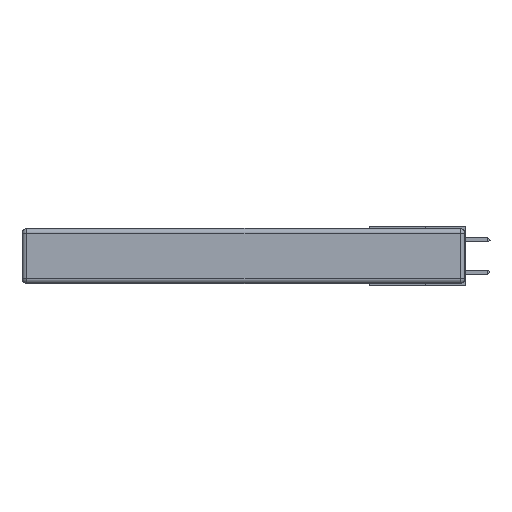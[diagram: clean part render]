
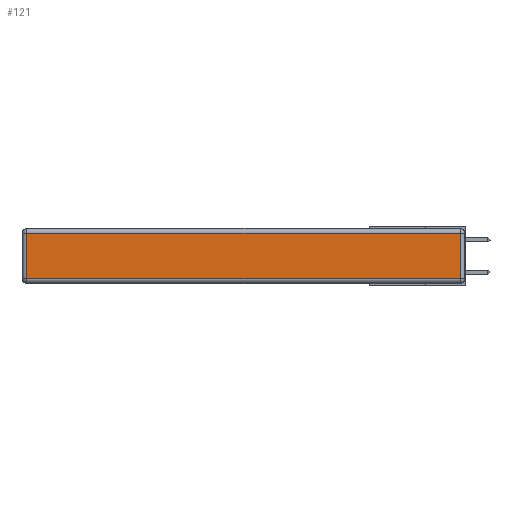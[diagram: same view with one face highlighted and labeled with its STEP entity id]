
A CAD part, left-side view. The second image highlights one B-rep face of the part: STEP entity #121.
In plain terms, the highlighted planar face has unit normal (-1, 0, 0).
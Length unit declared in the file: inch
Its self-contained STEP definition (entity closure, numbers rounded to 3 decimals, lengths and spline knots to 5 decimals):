
#121 = ADVANCED_FACE ( 'NONE', ( #670 ), #27151, .T. ) ;
#344 = VECTOR ( 'NONE', #29191, 39.37008 ) ;
#670 = FACE_OUTER_BOUND ( 'NONE', #27722, .T. ) ;
#856 = ORIENTED_EDGE ( 'NONE', *, *, #28431, .T. ) ;
#2791 = LINE ( 'NONE', #25806, #3155 ) ;
#3155 = VECTOR ( 'NONE', #28676, 39.37008 ) ;
#3933 = ORIENTED_EDGE ( 'NONE', *, *, #28927, .T. ) ;
#4337 = VERTEX_POINT ( 'NONE', #24066 ) ;
#5254 = CARTESIAN_POINT ( 'NONE',  ( 0., 2.72, -0.343 ) ) ;
#5694 = VECTOR ( 'NONE', #30632, 39.37008 ) ;
#6085 = VERTEX_POINT ( 'NONE', #6592 ) ;
#6592 = CARTESIAN_POINT ( 'NONE',  ( 0., 2.72, -0.03 ) ) ;
#6788 = CARTESIAN_POINT ( 'NONE',  ( 0., 0.03, -0.03 ) ) ;
#7111 = CARTESIAN_POINT ( 'NONE',  ( 0., 0., -0.343 ) ) ;
#13802 = VECTOR ( 'NONE', #24035, 39.37008 ) ;
#13983 = EDGE_CURVE ( 'NONE', #6085, #19820, #27896, .T. ) ;
#16495 = EDGE_CURVE ( 'NONE', #4337, #17255, #25729, .T. ) ;
#17074 = AXIS2_PLACEMENT_3D ( 'NONE', #7111, #26930, #17117 ) ;
#17117 = DIRECTION ( 'NONE',  ( 0., 0., 1. ) ) ;
#17255 = VERTEX_POINT ( 'NONE', #6788 ) ;
#19820 = VERTEX_POINT ( 'NONE', #32250 ) ;
#21319 = ORIENTED_EDGE ( 'NONE', *, *, #16495, .T. ) ;
#21330 = CARTESIAN_POINT ( 'NONE',  ( 0., 0., -0.313 ) ) ;
#24035 = DIRECTION ( 'NONE',  ( 0., -1., 0. ) ) ;
#24066 = CARTESIAN_POINT ( 'NONE',  ( 0., 0.03, -0.313 ) ) ;
#25358 = ORIENTED_EDGE ( 'NONE', *, *, #13983, .T. ) ;
#25729 = LINE ( 'NONE', #26883, #344 ) ;
#25806 = CARTESIAN_POINT ( 'NONE',  ( 0., 2.75, -0.03 ) ) ;
#26883 = CARTESIAN_POINT ( 'NONE',  ( 0., 0.03, -0.343 ) ) ;
#26930 = DIRECTION ( 'NONE',  ( -1., 0., 0. ) ) ;
#27151 = PLANE ( 'NONE',  #17074 ) ;
#27722 = EDGE_LOOP ( 'NONE', ( #3933, #21319, #856, #25358 ) ) ;
#27896 = LINE ( 'NONE', #5254, #5694 ) ;
#28431 = EDGE_CURVE ( 'NONE', #17255, #6085, #2791, .T. ) ;
#28676 = DIRECTION ( 'NONE',  ( 0., 1., 0. ) ) ;
#28927 = EDGE_CURVE ( 'NONE', #19820, #4337, #32093, .T. ) ;
#29191 = DIRECTION ( 'NONE',  ( 0., 0., 1. ) ) ;
#30632 = DIRECTION ( 'NONE',  ( 0., 0., -1. ) ) ;
#32093 = LINE ( 'NONE', #21330, #13802 ) ;
#32250 = CARTESIAN_POINT ( 'NONE',  ( 0., 2.72, -0.313 ) ) ;
